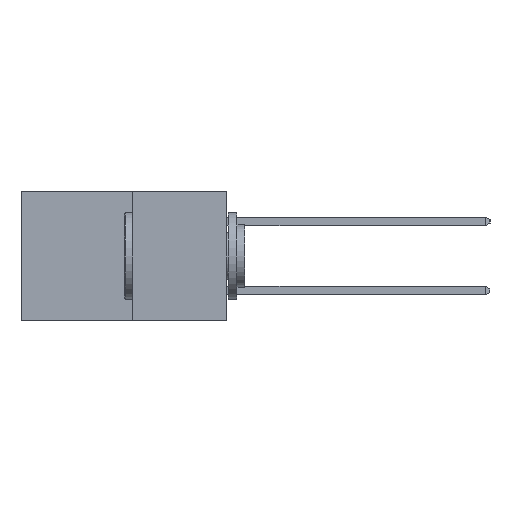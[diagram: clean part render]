
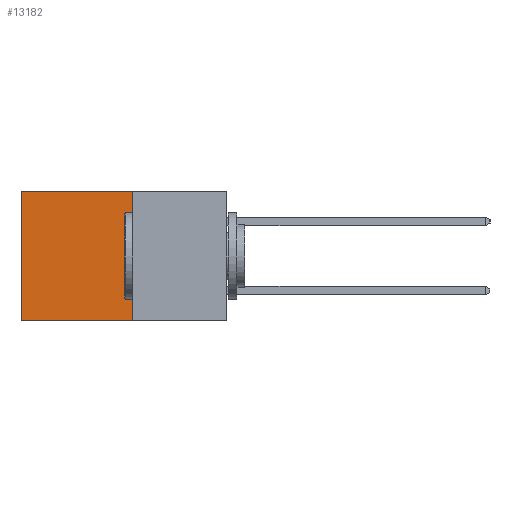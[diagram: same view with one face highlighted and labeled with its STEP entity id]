
A CAD part, left-side view. The second image highlights one B-rep face of the part: STEP entity #13182.
In plain terms, the highlighted planar face has unit normal (-1, 0, 0).
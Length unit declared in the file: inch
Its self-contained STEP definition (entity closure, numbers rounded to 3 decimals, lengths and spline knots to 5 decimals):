
#52 = CARTESIAN_POINT ( 'NONE',  ( 0.277, 0.27, 0. ) ) ;
#240 = VERTEX_POINT ( 'NONE', #10309 ) ;
#951 = DIRECTION ( 'NONE',  ( 1., 0., 0. ) ) ;
#1124 = EDGE_LOOP ( 'NONE', ( #10539, #13270, #8570, #13753 ) ) ;
#2763 = DIRECTION ( 'NONE',  ( 0., 1., 0. ) ) ;
#3000 = CARTESIAN_POINT ( 'NONE',  ( 0.277, 0.27, -0.37 ) ) ;
#3204 = CARTESIAN_POINT ( 'NONE',  ( 0.277, 0.27, -0.37 ) ) ;
#4925 = VECTOR ( 'NONE', #6071, 39.37008 ) ;
#5158 = VECTOR ( 'NONE', #12542, 39.37008 ) ;
#6071 = DIRECTION ( 'NONE',  ( 0., 1., 0. ) ) ;
#6197 = EDGE_CURVE ( 'NONE', #14527, #240, #17423, .T. ) ;
#6486 = VERTEX_POINT ( 'NONE', #11154 ) ;
#6613 = VECTOR ( 'NONE', #17306, 39.37008 ) ;
#8512 = AXIS2_PLACEMENT_3D ( 'NONE', #9055, #951, #10464 ) ;
#8570 = ORIENTED_EDGE ( 'NONE', *, *, #12101, .F. ) ;
#8775 = CARTESIAN_POINT ( 'NONE',  ( 0.277, 0.27, -0.37 ) ) ;
#9055 = CARTESIAN_POINT ( 'NONE',  ( 0.277, 0.27, -0.37 ) ) ;
#9619 = VECTOR ( 'NONE', #2763, 39.37008 ) ;
#10309 = CARTESIAN_POINT ( 'NONE',  ( 0.277, 0.59, -0.37 ) ) ;
#10464 = DIRECTION ( 'NONE',  ( 0., 0., -1. ) ) ;
#10539 = ORIENTED_EDGE ( 'NONE', *, *, #6197, .T. ) ;
#10551 = CARTESIAN_POINT ( 'NONE',  ( 0.277, 0.59, 0. ) ) ;
#11154 = CARTESIAN_POINT ( 'NONE',  ( 0.277, 0.27, 0. ) ) ;
#12016 = EDGE_CURVE ( 'NONE', #6486, #14527, #16439, .T. ) ;
#12101 = EDGE_CURVE ( 'NONE', #6486, #16057, #15184, .T. ) ;
#12315 = EDGE_CURVE ( 'NONE', #16057, #240, #15371, .T. ) ;
#12542 = DIRECTION ( 'NONE',  ( 0., 0., -1. ) ) ;
#13182 = ADVANCED_FACE ( 'NONE', ( #16597 ), #17228, .F. ) ;
#13270 = ORIENTED_EDGE ( 'NONE', *, *, #12315, .F. ) ;
#13753 = ORIENTED_EDGE ( 'NONE', *, *, #12016, .T. ) ;
#14527 = VERTEX_POINT ( 'NONE', #10551 ) ;
#15184 = LINE ( 'NONE', #3000, #5158 ) ;
#15371 = LINE ( 'NONE', #8775, #4925 ) ;
#15974 = CARTESIAN_POINT ( 'NONE',  ( 0.277, 0.59, -0.37 ) ) ;
#16057 = VERTEX_POINT ( 'NONE', #3204 ) ;
#16439 = LINE ( 'NONE', #52, #9619 ) ;
#16597 = FACE_OUTER_BOUND ( 'NONE', #1124, .T. ) ;
#17228 = PLANE ( 'NONE',  #8512 ) ;
#17306 = DIRECTION ( 'NONE',  ( 0., 0., -1. ) ) ;
#17423 = LINE ( 'NONE', #15974, #6613 ) ;
